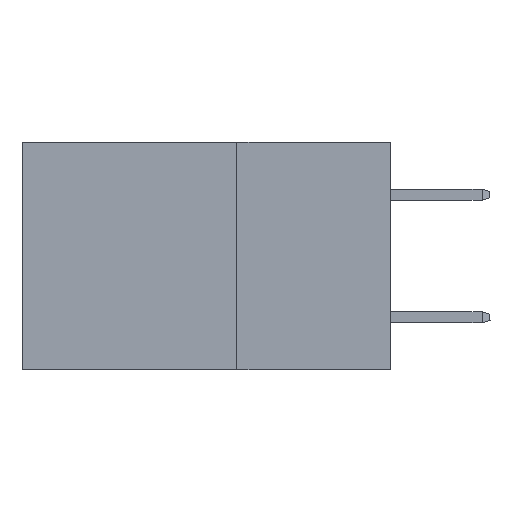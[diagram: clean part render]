
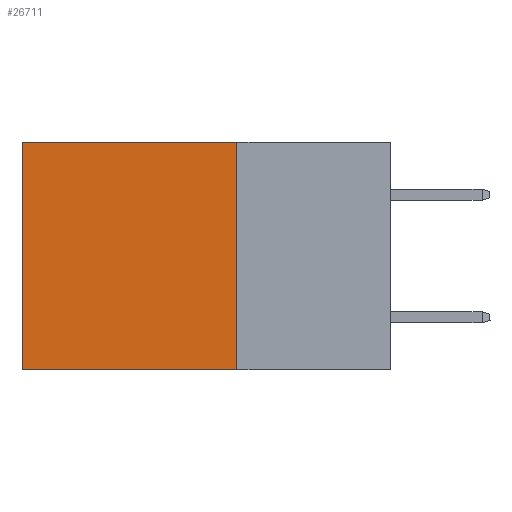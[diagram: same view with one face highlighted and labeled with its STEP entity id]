
A CAD part, left-side view. The second image highlights one B-rep face of the part: STEP entity #26711.
In plain terms, the highlighted planar face has unit normal (-1, 0, 0).
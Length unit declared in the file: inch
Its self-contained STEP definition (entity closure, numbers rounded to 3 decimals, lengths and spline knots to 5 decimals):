
#1463 = DIRECTION ( 'NONE',  ( 0., 0., -1. ) ) ;
#1598 = AXIS2_PLACEMENT_3D ( 'NONE', #15316, #4265, #1463 ) ;
#4265 = DIRECTION ( 'NONE',  ( 1., 0., 0. ) ) ;
#4694 = ORIENTED_EDGE ( 'NONE', *, *, #27964, .T. ) ;
#7668 = LINE ( 'NONE', #16824, #17761 ) ;
#11325 = CARTESIAN_POINT ( 'NONE',  ( 0.2875, 0.25, 0. ) ) ;
#11436 = DIRECTION ( 'NONE',  ( 0., 0., -1. ) ) ;
#12899 = VERTEX_POINT ( 'NONE', #34940 ) ;
#14341 = LINE ( 'NONE', #18393, #35830 ) ;
#14626 = VERTEX_POINT ( 'NONE', #24329 ) ;
#15316 = CARTESIAN_POINT ( 'NONE',  ( 0.2875, 0.25, 0. ) ) ;
#15688 = PLANE ( 'NONE',  #1598 ) ;
#16015 = EDGE_CURVE ( 'NONE', #21984, #12899, #14341, .T. ) ;
#16485 = ORIENTED_EDGE ( 'NONE', *, *, #26370, .T. ) ;
#16765 = LINE ( 'NONE', #34713, #29884 ) ;
#16824 = CARTESIAN_POINT ( 'NONE',  ( 0.2875, 0.6, 0. ) ) ;
#17720 = ORIENTED_EDGE ( 'NONE', *, *, #34141, .F. ) ;
#17761 = VECTOR ( 'NONE', #11436, 39.37008 ) ;
#18056 = DIRECTION ( 'NONE',  ( 0., 1., 0. ) ) ;
#18393 = CARTESIAN_POINT ( 'NONE',  ( 0.2875, 0.25, -0.37 ) ) ;
#19117 = DIRECTION ( 'NONE',  ( 0., 1., 0. ) ) ;
#19415 = CARTESIAN_POINT ( 'NONE',  ( 0.2875, 0.25, 0. ) ) ;
#21984 = VERTEX_POINT ( 'NONE', #26935 ) ;
#22112 = DIRECTION ( 'NONE',  ( 0., 0., -1. ) ) ;
#24172 = VERTEX_POINT ( 'NONE', #11325 ) ;
#24329 = CARTESIAN_POINT ( 'NONE',  ( 0.2875, 0.6, 0. ) ) ;
#26370 = EDGE_CURVE ( 'NONE', #14626, #12899, #7668, .T. ) ;
#26711 = ADVANCED_FACE ( 'NONE', ( #29961 ), #15688, .F. ) ;
#26935 = CARTESIAN_POINT ( 'NONE',  ( 0.2875, 0.25, -0.37 ) ) ;
#27964 = EDGE_CURVE ( 'NONE', #24172, #14626, #16765, .T. ) ;
#28147 = LINE ( 'NONE', #19415, #28581 ) ;
#28581 = VECTOR ( 'NONE', #22112, 39.37008 ) ;
#28809 = ORIENTED_EDGE ( 'NONE', *, *, #16015, .F. ) ;
#29884 = VECTOR ( 'NONE', #18056, 39.37008 ) ;
#29961 = FACE_OUTER_BOUND ( 'NONE', #36124, .T. ) ;
#34141 = EDGE_CURVE ( 'NONE', #24172, #21984, #28147, .T. ) ;
#34713 = CARTESIAN_POINT ( 'NONE',  ( 0.2875, 0.25, 0. ) ) ;
#34940 = CARTESIAN_POINT ( 'NONE',  ( 0.2875, 0.6, -0.37 ) ) ;
#35830 = VECTOR ( 'NONE', #19117, 39.37008 ) ;
#36124 = EDGE_LOOP ( 'NONE', ( #16485, #28809, #17720, #4694 ) ) ;
